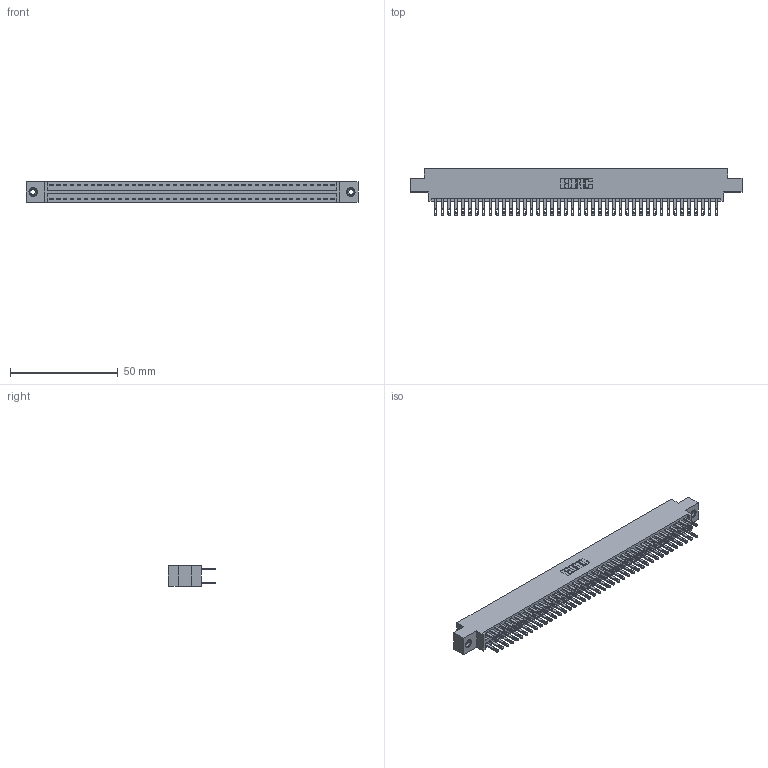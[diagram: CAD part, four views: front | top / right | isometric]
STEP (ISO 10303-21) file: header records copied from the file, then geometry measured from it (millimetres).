
FILE_DESCRIPTION (( 'STEP AP203' ), '1' );
FILE_NAME ('896-084-500-808.STEP', '2021-07-28T02:28:02', ( '' ), ( '' ), 'SwSTEP 2.0', 'SolidWorks 2020', '' );
FILE_SCHEMA (( 'CONFIG_CONTROL_DESIGN' ));
Length unit declared in the file: inch
Products named in the file (4): 345-250-001_345-250-003-102; 345-292-001_345-293-100; 896-084-500-808; 846 Part_0.170 Offset - 0.156 Dia-TI
Assembly tree (87 placements, depth 2):
  896-084-500-808
    846 Part_0.170 Offset - 0.156 Dia-TI
    345-292-001_345-293-100  x84
    345-250-001_345-250-003-102  x2
Bounding box: 153.92 x 21.84 x 9.4 mm (x, y, z)
Volume: 15105.1 mm3; surface area: 21841.8 mm2
Topology: 87 solids, 87 shells, 4218 faces, 12825 edges, 8542 vertices
Faces by surface type: plane 2548, cylinder 1654, cone 12, torus 4
Entity records: 28658 total; most frequent: CARTESIAN_POINT 4707, ORIENTED_EDGE 4634, DIRECTION 4227, EDGE_CURVE 2317, VECTOR 1993, LINE 1993, VERTEX_POINT 1540, AXIS2_PLACEMENT_3D 1117
